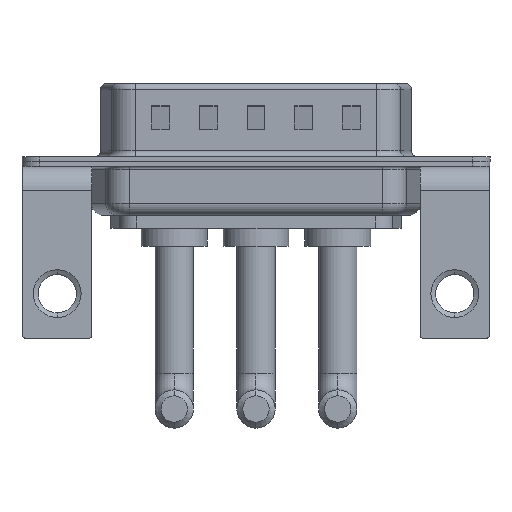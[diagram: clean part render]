
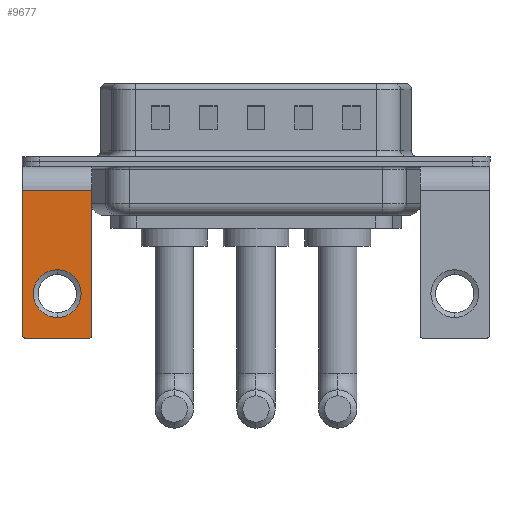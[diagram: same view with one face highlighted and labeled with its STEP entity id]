
A CAD part, front view. The second image highlights one B-rep face of the part: STEP entity #9677.
In plain terms, the highlighted planar face has unit normal (0, -1, 0).
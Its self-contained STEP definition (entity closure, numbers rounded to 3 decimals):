
#237 = AXIS2_PLACEMENT_3D ( 'NONE', #4552, #12551, #1087 ) ;
#286 = DIRECTION ( 'NONE',  ( 0., 1., 0. ) ) ;
#883 = CARTESIAN_POINT ( 'NONE',  ( 0., -6.25, -9.07 ) ) ;
#929 = EDGE_CURVE ( 'NONE', #6358, #13877, #13300, .T. ) ;
#1087 = DIRECTION ( 'NONE',  ( 0., 0., 1. ) ) ;
#1746 = CARTESIAN_POINT ( 'NONE',  ( -2.9, -6.25, -14.55 ) ) ;
#1759 = CARTESIAN_POINT ( 'NONE',  ( -2.65, -6.25, -14.8 ) ) ;
#1934 = EDGE_LOOP ( 'NONE', ( #12482, #4787, #15826, #14261, #8670, #7531 ) ) ;
#2039 = EDGE_CURVE ( 'NONE', #10893, #2095, #12565, .T. ) ;
#2095 = VERTEX_POINT ( 'NONE', #8314 ) ;
#2228 = CARTESIAN_POINT ( 'NONE',  ( 2.9, -6.25, -2.4 ) ) ;
#2302 = DIRECTION ( 'NONE',  ( 0., 1., 0. ) ) ;
#2365 = DIRECTION ( 'NONE',  ( -1., 0., 0. ) ) ;
#2446 = CARTESIAN_POINT ( 'NONE',  ( 2.9, -6.25, -2.4 ) ) ;
#2830 = CARTESIAN_POINT ( 'NONE',  ( 2.65, -6.25, -14.8 ) ) ;
#2936 = CARTESIAN_POINT ( 'NONE',  ( -2.9, -6.25, -2.4 ) ) ;
#3011 = VERTEX_POINT ( 'NONE', #1759 ) ;
#3175 = CARTESIAN_POINT ( 'NONE',  ( 0., -6.25, -13.07 ) ) ;
#3249 = VECTOR ( 'NONE', #13321, 1000. ) ;
#3856 = EDGE_CURVE ( 'NONE', #6992, #3011, #12338, .T. ) ;
#3919 = ORIENTED_EDGE ( 'NONE', *, *, #11066, .T. ) ;
#3940 = AXIS2_PLACEMENT_3D ( 'NONE', #7569, #12719, #15343 ) ;
#4552 = CARTESIAN_POINT ( 'NONE',  ( -2.65, -6.25, -14.55 ) ) ;
#4787 = ORIENTED_EDGE ( 'NONE', *, *, #3856, .T. ) ;
#4966 = AXIS2_PLACEMENT_3D ( 'NONE', #13885, #7194, #7448 ) ;
#6161 = PLANE ( 'NONE',  #13793 ) ;
#6358 = VERTEX_POINT ( 'NONE', #883 ) ;
#6380 = EDGE_CURVE ( 'NONE', #10893, #9428, #13787, .T. ) ;
#6992 = VERTEX_POINT ( 'NONE', #1746 ) ;
#7040 = EDGE_CURVE ( 'NONE', #7464, #3011, #11775, .T. ) ;
#7177 = DIRECTION ( 'NONE',  ( 0., 0., 1. ) ) ;
#7194 = DIRECTION ( 'NONE',  ( 0., 1., 0. ) ) ;
#7448 = DIRECTION ( 'NONE',  ( 0., 0., 1. ) ) ;
#7464 = VERTEX_POINT ( 'NONE', #2830 ) ;
#7531 = ORIENTED_EDGE ( 'NONE', *, *, #2039, .T. ) ;
#7569 = CARTESIAN_POINT ( 'NONE',  ( 2.65, -6.25, -14.55 ) ) ;
#7900 = DIRECTION ( 'NONE',  ( 0., 0., -1. ) ) ;
#8037 = CARTESIAN_POINT ( 'NONE',  ( 0., -6.25, -11.07 ) ) ;
#8314 = CARTESIAN_POINT ( 'NONE',  ( -2.9, -6.25, -2.4 ) ) ;
#8670 = ORIENTED_EDGE ( 'NONE', *, *, #6380, .F. ) ;
#8766 = VECTOR ( 'NONE', #7900, 1000. ) ;
#9293 = CIRCLE ( 'NONE', #3940, 0.25 ) ;
#9428 = VERTEX_POINT ( 'NONE', #12849 ) ;
#9677 = ADVANCED_FACE ( 'NONE', ( #14960, #11232 ), #6161, .F. ) ;
#10088 = DIRECTION ( 'NONE',  ( 0., 0., 1. ) ) ;
#10425 = LINE ( 'NONE', #2936, #8766 ) ;
#10893 = VERTEX_POINT ( 'NONE', #13476 ) ;
#11066 = EDGE_CURVE ( 'NONE', #13877, #6358, #14042, .T. ) ;
#11232 = FACE_OUTER_BOUND ( 'NONE', #1934, .T. ) ;
#11240 = DIRECTION ( 'NONE',  ( 0., 0., -1. ) ) ;
#11305 = CARTESIAN_POINT ( 'NONE',  ( 2.9, -6.25, -2.4 ) ) ;
#11775 = LINE ( 'NONE', #15843, #3249 ) ;
#12283 = ORIENTED_EDGE ( 'NONE', *, *, #929, .T. ) ;
#12338 = CIRCLE ( 'NONE', #237, 0.25 ) ;
#12482 = ORIENTED_EDGE ( 'NONE', *, *, #16412, .T. ) ;
#12551 = DIRECTION ( 'NONE',  ( 0., -1., 0. ) ) ;
#12565 = LINE ( 'NONE', #2446, #15493 ) ;
#12719 = DIRECTION ( 'NONE',  ( 0., -1., 0. ) ) ;
#12849 = CARTESIAN_POINT ( 'NONE',  ( 2.9, -6.25, -14.55 ) ) ;
#13300 = CIRCLE ( 'NONE', #4966, 2. ) ;
#13321 = DIRECTION ( 'NONE',  ( -1., 0., 0. ) ) ;
#13476 = CARTESIAN_POINT ( 'NONE',  ( 2.9, -6.25, -2.4 ) ) ;
#13660 = EDGE_LOOP ( 'NONE', ( #3919, #12283 ) ) ;
#13787 = LINE ( 'NONE', #2228, #14907 ) ;
#13793 = AXIS2_PLACEMENT_3D ( 'NONE', #11305, #2302, #7177 ) ;
#13877 = VERTEX_POINT ( 'NONE', #3175 ) ;
#13885 = CARTESIAN_POINT ( 'NONE',  ( 0., -6.25, -11.07 ) ) ;
#14042 = CIRCLE ( 'NONE', #16171, 2. ) ;
#14261 = ORIENTED_EDGE ( 'NONE', *, *, #15185, .T. ) ;
#14907 = VECTOR ( 'NONE', #11240, 1000. ) ;
#14960 = FACE_BOUND ( 'NONE', #13660, .T. ) ;
#15185 = EDGE_CURVE ( 'NONE', #7464, #9428, #9293, .T. ) ;
#15343 = DIRECTION ( 'NONE',  ( 0., 0., 1. ) ) ;
#15493 = VECTOR ( 'NONE', #2365, 1000. ) ;
#15826 = ORIENTED_EDGE ( 'NONE', *, *, #7040, .F. ) ;
#15843 = CARTESIAN_POINT ( 'NONE',  ( 2.9, -6.25, -14.8 ) ) ;
#16171 = AXIS2_PLACEMENT_3D ( 'NONE', #8037, #286, #10088 ) ;
#16412 = EDGE_CURVE ( 'NONE', #2095, #6992, #10425, .T. ) ;
